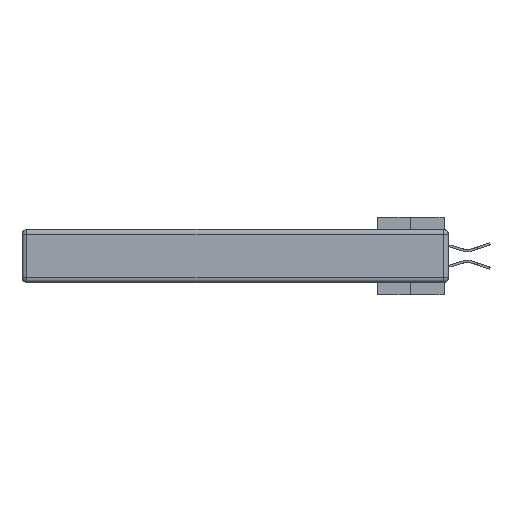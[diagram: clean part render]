
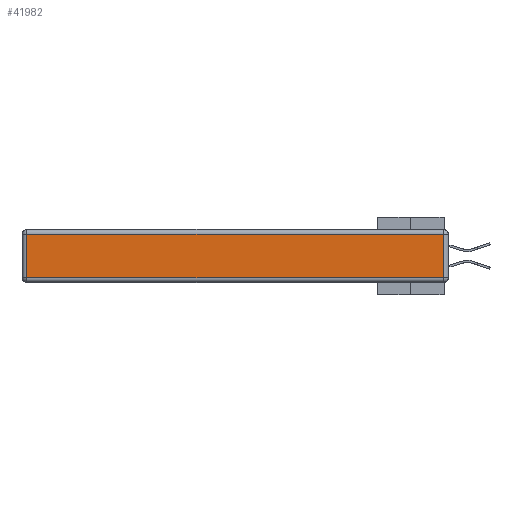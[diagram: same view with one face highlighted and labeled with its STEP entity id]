
A CAD part, left-side view. The second image highlights one B-rep face of the part: STEP entity #41982.
In plain terms, the highlighted planar face has unit normal (-1, 0, 0).
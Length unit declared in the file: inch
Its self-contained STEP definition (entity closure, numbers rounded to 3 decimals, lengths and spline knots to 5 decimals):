
#6162 = LINE ( 'NONE', #31746, #25881 ) ;
#7009 = CARTESIAN_POINT ( 'NONE',  ( 0., 2.72, -0.03 ) ) ;
#9150 = AXIS2_PLACEMENT_3D ( 'NONE', #31963, #9814, #24716 ) ;
#9389 = CARTESIAN_POINT ( 'NONE',  ( 0., 2.75, -0.03 ) ) ;
#9814 = DIRECTION ( 'NONE',  ( -1., 0., 0. ) ) ;
#10636 = CARTESIAN_POINT ( 'NONE',  ( 0., 0.03, -0.313 ) ) ;
#11605 = VERTEX_POINT ( 'NONE', #17602 ) ;
#17602 = CARTESIAN_POINT ( 'NONE',  ( 0., 2.72, -0.313 ) ) ;
#18072 = LINE ( 'NONE', #9389, #38904 ) ;
#18392 = EDGE_CURVE ( 'NONE', #11605, #23539, #47176, .T. ) ;
#20091 = DIRECTION ( 'NONE',  ( 0., 1., 0. ) ) ;
#20861 = LINE ( 'NONE', #37360, #23206 ) ;
#20906 = EDGE_CURVE ( 'NONE', #37288, #33239, #18072, .T. ) ;
#21153 = ORIENTED_EDGE ( 'NONE', *, *, #20906, .T. ) ;
#21526 = ORIENTED_EDGE ( 'NONE', *, *, #40759, .T. ) ;
#21913 = EDGE_CURVE ( 'NONE', #33239, #11605, #20861, .T. ) ;
#23206 = VECTOR ( 'NONE', #23414, 39.37008 ) ;
#23414 = DIRECTION ( 'NONE',  ( 0., 0., -1. ) ) ;
#23539 = VERTEX_POINT ( 'NONE', #10636 ) ;
#24716 = DIRECTION ( 'NONE',  ( 0., 0., 1. ) ) ;
#24813 = DIRECTION ( 'NONE',  ( 0., 0., 1. ) ) ;
#25881 = VECTOR ( 'NONE', #24813, 39.37008 ) ;
#26108 = CARTESIAN_POINT ( 'NONE',  ( 0., 0.03, -0.03 ) ) ;
#28004 = EDGE_LOOP ( 'NONE', ( #46669, #21526, #21153, #34691 ) ) ;
#29964 = CARTESIAN_POINT ( 'NONE',  ( 0., 0., -0.313 ) ) ;
#31746 = CARTESIAN_POINT ( 'NONE',  ( 0., 0.03, -0.343 ) ) ;
#31963 = CARTESIAN_POINT ( 'NONE',  ( 0., 0., -0.343 ) ) ;
#33239 = VERTEX_POINT ( 'NONE', #7009 ) ;
#34691 = ORIENTED_EDGE ( 'NONE', *, *, #21913, .T. ) ;
#37288 = VERTEX_POINT ( 'NONE', #26108 ) ;
#37360 = CARTESIAN_POINT ( 'NONE',  ( 0., 2.72, -0.343 ) ) ;
#37399 = VECTOR ( 'NONE', #37739, 39.37008 ) ;
#37739 = DIRECTION ( 'NONE',  ( 0., -1., 0. ) ) ;
#38904 = VECTOR ( 'NONE', #20091, 39.37008 ) ;
#40759 = EDGE_CURVE ( 'NONE', #23539, #37288, #6162, .T. ) ;
#41047 = FACE_OUTER_BOUND ( 'NONE', #28004, .T. ) ;
#41982 = ADVANCED_FACE ( 'NONE', ( #41047 ), #46986, .T. ) ;
#46669 = ORIENTED_EDGE ( 'NONE', *, *, #18392, .T. ) ;
#46986 = PLANE ( 'NONE',  #9150 ) ;
#47176 = LINE ( 'NONE', #29964, #37399 ) ;
